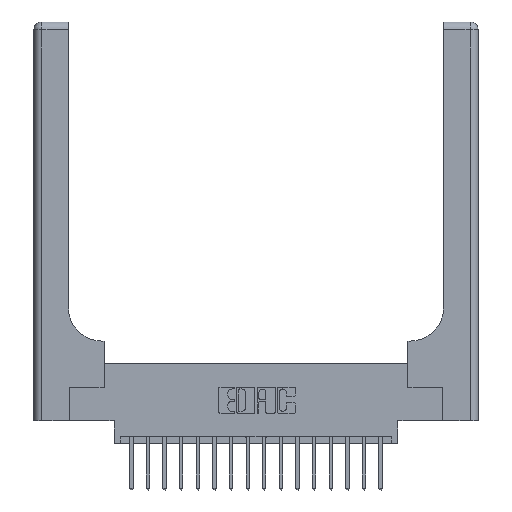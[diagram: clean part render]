
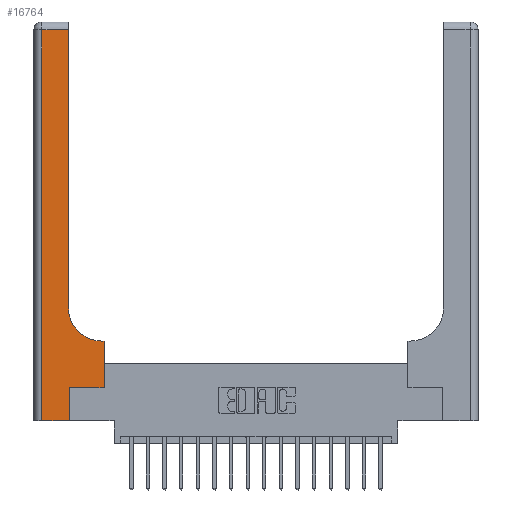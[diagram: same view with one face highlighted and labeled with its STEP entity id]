
A CAD part, top view. The second image highlights one B-rep face of the part: STEP entity #16764.
In plain terms, the highlighted planar face has unit normal (0, 0, 1).
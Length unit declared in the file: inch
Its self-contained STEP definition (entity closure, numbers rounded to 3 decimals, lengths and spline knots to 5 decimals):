
#298 = EDGE_CURVE ( 'NONE', #11549, #11642, #3889, .T. ) ;
#898 = ORIENTED_EDGE ( 'NONE', *, *, #18647, .T. ) ;
#919 = ORIENTED_EDGE ( 'NONE', *, *, #18084, .T. ) ;
#1045 = ORIENTED_EDGE ( 'NONE', *, *, #8081, .T. ) ;
#1303 = VERTEX_POINT ( 'NONE', #12566 ) ;
#1403 = DIRECTION ( 'NONE',  ( 0., 0., -1. ) ) ;
#1740 = CARTESIAN_POINT ( 'NONE',  ( 0.26, 3., 0.37 ) ) ;
#2223 = CARTESIAN_POINT ( 'NONE',  ( 0.528, 0.25, 0.37 ) ) ;
#2301 = LINE ( 'NONE', #15869, #14907 ) ;
#2386 = CIRCLE ( 'NONE', #3991, 0.25 ) ;
#2763 = LINE ( 'NONE', #7162, #8871 ) ;
#3606 = DIRECTION ( 'NONE',  ( 0., -1., 0. ) ) ;
#3717 = DIRECTION ( 'NONE',  ( 0., 1., 0. ) ) ;
#3889 = LINE ( 'NONE', #9968, #14131 ) ;
#3991 = AXIS2_PLACEMENT_3D ( 'NONE', #13019, #8340, #19103 ) ;
#4168 = ORIENTED_EDGE ( 'NONE', *, *, #7705, .T. ) ;
#4771 = ORIENTED_EDGE ( 'NONE', *, *, #9605, .T. ) ;
#6027 = FACE_OUTER_BOUND ( 'NONE', #11729, .T. ) ;
#6251 = DIRECTION ( 'NONE',  ( 0., 1., 0. ) ) ;
#6285 = AXIS2_PLACEMENT_3D ( 'NONE', #15075, #1403, #13590 ) ;
#6370 = EDGE_CURVE ( 'NONE', #7736, #15305, #11211, .T. ) ;
#6620 = VECTOR ( 'NONE', #16149, 39.37008 ) ;
#7162 = CARTESIAN_POINT ( 'NONE',  ( 0., 0., 0.37 ) ) ;
#7285 = LINE ( 'NONE', #13364, #19033 ) ;
#7310 = DIRECTION ( 'NONE',  ( -1., 0., 0. ) ) ;
#7705 = EDGE_CURVE ( 'NONE', #15305, #9786, #14871, .T. ) ;
#7736 = VERTEX_POINT ( 'NONE', #10001 ) ;
#8081 = EDGE_CURVE ( 'NONE', #14151, #7736, #10063, .T. ) ;
#8340 = DIRECTION ( 'NONE',  ( 0., 0., -1. ) ) ;
#8576 = CARTESIAN_POINT ( 'NONE',  ( 0.06, 2.94, 0.37 ) ) ;
#8871 = VECTOR ( 'NONE', #10353, 39.37008 ) ;
#9493 = EDGE_CURVE ( 'NONE', #1303, #11549, #16698, .T. ) ;
#9605 = EDGE_CURVE ( 'NONE', #9786, #1303, #2386, .T. ) ;
#9786 = VERTEX_POINT ( 'NONE', #18389 ) ;
#9968 = CARTESIAN_POINT ( 'NONE',  ( 0., 2.94, 0.37 ) ) ;
#10001 = CARTESIAN_POINT ( 'NONE',  ( 0.528, 0.25, 0.37 ) ) ;
#10063 = LINE ( 'NONE', #19350, #6620 ) ;
#10353 = DIRECTION ( 'NONE',  ( 1., 0., 0. ) ) ;
#10790 = PLANE ( 'NONE',  #6285 ) ;
#11103 = CARTESIAN_POINT ( 'NONE',  ( 0.528, 0.6, 0.37 ) ) ;
#11211 = LINE ( 'NONE', #2223, #12148 ) ;
#11242 = ORIENTED_EDGE ( 'NONE', *, *, #298, .T. ) ;
#11488 = DIRECTION ( 'NONE',  ( 0., 1., 0. ) ) ;
#11549 = VERTEX_POINT ( 'NONE', #15956 ) ;
#11642 = VERTEX_POINT ( 'NONE', #8576 ) ;
#11679 = CARTESIAN_POINT ( 'NONE',  ( 0.265, 0.25, 0.37 ) ) ;
#11729 = EDGE_LOOP ( 'NONE', ( #13690, #11242, #919, #898, #12158, #1045, #15908, #4168, #4771 ) ) ;
#12148 = VECTOR ( 'NONE', #3717, 39.37008 ) ;
#12158 = ORIENTED_EDGE ( 'NONE', *, *, #17071, .T. ) ;
#12566 = CARTESIAN_POINT ( 'NONE',  ( 0.26, 0.85, 0.37 ) ) ;
#13005 = CARTESIAN_POINT ( 'NONE',  ( 0.26, 0.6, 0.37 ) ) ;
#13019 = CARTESIAN_POINT ( 'NONE',  ( 0.51, 0.85, 0.37 ) ) ;
#13364 = CARTESIAN_POINT ( 'NONE',  ( 0.265, 0., 0.37 ) ) ;
#13590 = DIRECTION ( 'NONE',  ( -1., 0., 0. ) ) ;
#13690 = ORIENTED_EDGE ( 'NONE', *, *, #9493, .T. ) ;
#13785 = VERTEX_POINT ( 'NONE', #16665 ) ;
#14131 = VECTOR ( 'NONE', #16046, 39.37008 ) ;
#14151 = VERTEX_POINT ( 'NONE', #11679 ) ;
#14271 = CARTESIAN_POINT ( 'NONE',  ( 0.265, 0., 0.37 ) ) ;
#14813 = VECTOR ( 'NONE', #7310, 39.37008 ) ;
#14871 = LINE ( 'NONE', #13005, #14813 ) ;
#14907 = VECTOR ( 'NONE', #3606, 39.37008 ) ;
#15075 = CARTESIAN_POINT ( 'NONE',  ( 0., 3., 0.37 ) ) ;
#15305 = VERTEX_POINT ( 'NONE', #11103 ) ;
#15869 = CARTESIAN_POINT ( 'NONE',  ( 0.06, 3., 0.37 ) ) ;
#15908 = ORIENTED_EDGE ( 'NONE', *, *, #6370, .T. ) ;
#15956 = CARTESIAN_POINT ( 'NONE',  ( 0.26, 2.94, 0.37 ) ) ;
#16046 = DIRECTION ( 'NONE',  ( -1., 0., 0. ) ) ;
#16149 = DIRECTION ( 'NONE',  ( 1., 0., 0. ) ) ;
#16665 = CARTESIAN_POINT ( 'NONE',  ( 0.06, 0., 0.37 ) ) ;
#16698 = LINE ( 'NONE', #1740, #18635 ) ;
#16764 = ADVANCED_FACE ( 'NONE', ( #6027 ), #10790, .F. ) ;
#16915 = VERTEX_POINT ( 'NONE', #14271 ) ;
#17071 = EDGE_CURVE ( 'NONE', #16915, #14151, #7285, .T. ) ;
#18084 = EDGE_CURVE ( 'NONE', #11642, #13785, #2301, .T. ) ;
#18389 = CARTESIAN_POINT ( 'NONE',  ( 0.51, 0.6, 0.37 ) ) ;
#18635 = VECTOR ( 'NONE', #6251, 39.37008 ) ;
#18647 = EDGE_CURVE ( 'NONE', #13785, #16915, #2763, .T. ) ;
#19033 = VECTOR ( 'NONE', #11488, 39.37008 ) ;
#19103 = DIRECTION ( 'NONE',  ( 1., 0., 0. ) ) ;
#19350 = CARTESIAN_POINT ( 'NONE',  ( 0.265, 0.25, 0.37 ) ) ;
